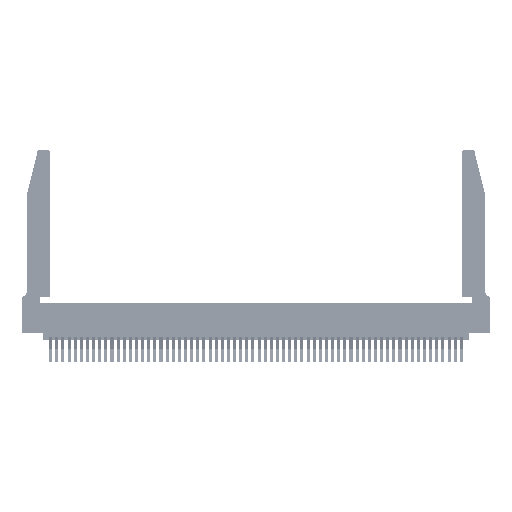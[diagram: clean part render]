
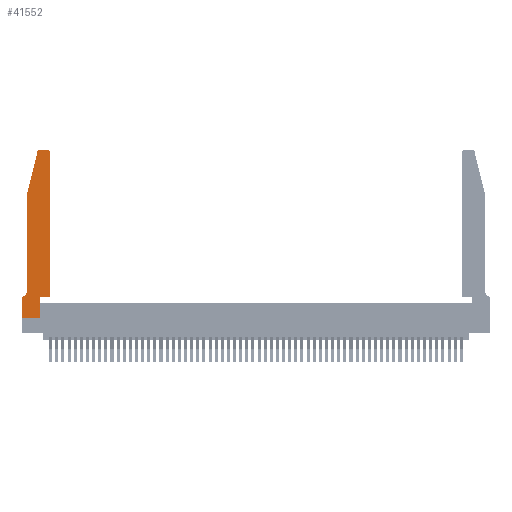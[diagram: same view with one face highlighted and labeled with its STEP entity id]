
A CAD part, top view. The second image highlights one B-rep face of the part: STEP entity #41552.
In plain terms, the highlighted planar face has unit normal (0, 0, 1).
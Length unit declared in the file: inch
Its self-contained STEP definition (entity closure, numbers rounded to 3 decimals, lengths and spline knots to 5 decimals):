
#506 = ORIENTED_EDGE ( 'NONE', *, *, #52466, .T. ) ;
#1064 = CARTESIAN_POINT ( 'NONE',  ( 0.284, 2.72, 0.37 ) ) ;
#1085 = AXIS2_PLACEMENT_3D ( 'NONE', #30913, #9419, #38880 ) ;
#1882 = DIRECTION ( 'NONE',  ( 0., -1., 0. ) ) ;
#2867 = VERTEX_POINT ( 'NONE', #22507 ) ;
#3102 = VERTEX_POINT ( 'NONE', #41610 ) ;
#3352 = DIRECTION ( 'NONE',  ( 0., 1., 0. ) ) ;
#3714 = VERTEX_POINT ( 'NONE', #50578 ) ;
#4692 = CARTESIAN_POINT ( 'NONE',  ( 0.4505, 0.35, 0.37 ) ) ;
#4721 = CARTESIAN_POINT ( 'NONE',  ( 0.2605, 2.75, 0.37 ) ) ;
#5341 = DIRECTION ( 'NONE',  ( 0., 0., 1. ) ) ;
#5504 = VECTOR ( 'NONE', #34674, 39.37008 ) ;
#6053 = ORIENTED_EDGE ( 'NONE', *, *, #23268, .T. ) ;
#6073 = CARTESIAN_POINT ( 'NONE',  ( 0.4205, 2.75, 0.37 ) ) ;
#6304 = VERTEX_POINT ( 'NONE', #43441 ) ;
#6562 = LINE ( 'NONE', #4721, #50968 ) ;
#6827 = LINE ( 'NONE', #18709, #5504 ) ;
#8562 = VERTEX_POINT ( 'NONE', #16446 ) ;
#9251 = LINE ( 'NONE', #15184, #30469 ) ;
#9419 = DIRECTION ( 'NONE',  ( 0., 0., 1. ) ) ;
#9603 = VERTEX_POINT ( 'NONE', #38207 ) ;
#9694 = EDGE_CURVE ( 'NONE', #6304, #2867, #43880, .T. ) ;
#10187 = CARTESIAN_POINT ( 'NONE',  ( 0., 0., 0.37 ) ) ;
#10764 = EDGE_CURVE ( 'NONE', #15551, #9603, #6562, .T. ) ;
#10932 = CIRCLE ( 'NONE', #53073, 0.07 ) ;
#10985 = DIRECTION ( 'NONE',  ( 1., 0., 0. ) ) ;
#11392 = DIRECTION ( 'NONE',  ( -1., 0., 0. ) ) ;
#11738 = CARTESIAN_POINT ( 'NONE',  ( 0.0055, 0.42, 0.37 ) ) ;
#12005 = VECTOR ( 'NONE', #18521, 39.37008 ) ;
#12232 = ORIENTED_EDGE ( 'NONE', *, *, #9694, .T. ) ;
#13826 = ORIENTED_EDGE ( 'NONE', *, *, #10764, .T. ) ;
#13906 = EDGE_CURVE ( 'NONE', #50789, #3714, #10932, .T. ) ;
#14759 = ORIENTED_EDGE ( 'NONE', *, *, #17824, .T. ) ;
#14762 = FACE_OUTER_BOUND ( 'NONE', #15753, .T. ) ;
#14810 = CARTESIAN_POINT ( 'NONE',  ( 0.0755, 0.42, 0.37 ) ) ;
#15184 = CARTESIAN_POINT ( 'NONE',  ( 0.2865, 0.35, 0.37 ) ) ;
#15551 = VERTEX_POINT ( 'NONE', #6073 ) ;
#15753 = EDGE_LOOP ( 'NONE', ( #13826, #19654, #27591, #53457, #26829, #46056, #14759, #12232, #38627, #6053, #506, #33454 ) ) ;
#15930 = VECTOR ( 'NONE', #34876, 39.37008 ) ;
#16446 = CARTESIAN_POINT ( 'NONE',  ( 0.25487, 2.72718, 0.37 ) ) ;
#16465 = AXIS2_PLACEMENT_3D ( 'NONE', #1064, #5341, #35334 ) ;
#17552 = PLANE ( 'NONE',  #1085 ) ;
#17824 = EDGE_CURVE ( 'NONE', #42799, #6304, #25802, .T. ) ;
#17962 = VECTOR ( 'NONE', #1882, 39.37008 ) ;
#18521 = DIRECTION ( 'NONE',  ( 1., 0., 0. ) ) ;
#18709 = CARTESIAN_POINT ( 'NONE',  ( 0.0755, 0.35, 0.37 ) ) ;
#19654 = ORIENTED_EDGE ( 'NONE', *, *, #48358, .T. ) ;
#21516 = VECTOR ( 'NONE', #36218, 39.37008 ) ;
#22507 = CARTESIAN_POINT ( 'NONE',  ( 0.2865, 0., 0.37 ) ) ;
#23268 = EDGE_CURVE ( 'NONE', #35293, #23923, #53949, .T. ) ;
#23913 = EDGE_CURVE ( 'NONE', #3102, #15551, #49177, .T. ) ;
#23923 = VERTEX_POINT ( 'NONE', #40965 ) ;
#25242 = LINE ( 'NONE', #4692, #15930 ) ;
#25802 = LINE ( 'NONE', #28929, #41071 ) ;
#26232 = EDGE_CURVE ( 'NONE', #36796, #50789, #54436, .T. ) ;
#26829 = ORIENTED_EDGE ( 'NONE', *, *, #13906, .T. ) ;
#27591 = ORIENTED_EDGE ( 'NONE', *, *, #48375, .T. ) ;
#28174 = DIRECTION ( 'NONE',  ( 0., 0., 1. ) ) ;
#28278 = DIRECTION ( 'NONE',  ( 0., 0., -1. ) ) ;
#28599 = AXIS2_PLACEMENT_3D ( 'NONE', #49247, #28174, #36506 ) ;
#28660 = CARTESIAN_POINT ( 'NONE',  ( 0.2865, 0.35, 0.37 ) ) ;
#28929 = CARTESIAN_POINT ( 'NONE',  ( 0., 0., 0.37 ) ) ;
#30469 = VECTOR ( 'NONE', #3352, 39.37008 ) ;
#30913 = CARTESIAN_POINT ( 'NONE',  ( 0., 0.35, 0.37 ) ) ;
#32322 = CARTESIAN_POINT ( 'NONE',  ( 0.4505, 0.35, 0.37 ) ) ;
#32751 = VECTOR ( 'NONE', #10985, 39.37008 ) ;
#32819 = LINE ( 'NONE', #38860, #21516 ) ;
#33454 = ORIENTED_EDGE ( 'NONE', *, *, #23913, .T. ) ;
#34516 = CARTESIAN_POINT ( 'NONE',  ( 0., 0.35, 0.37 ) ) ;
#34674 = DIRECTION ( 'NONE',  ( -1., 0., 0. ) ) ;
#34876 = DIRECTION ( 'NONE',  ( 0., 1., 0. ) ) ;
#35293 = VERTEX_POINT ( 'NONE', #28660 ) ;
#35334 = DIRECTION ( 'NONE',  ( 1., 0., 0. ) ) ;
#36218 = DIRECTION ( 'NONE',  ( -0.239, -0.971, 0. ) ) ;
#36506 = DIRECTION ( 'NONE',  ( 1., 0., 0. ) ) ;
#36528 = CARTESIAN_POINT ( 'NONE',  ( 0.0755, 2., 0.37 ) ) ;
#36796 = VERTEX_POINT ( 'NONE', #50878 ) ;
#38207 = CARTESIAN_POINT ( 'NONE',  ( 0.284, 2.75, 0.37 ) ) ;
#38627 = ORIENTED_EDGE ( 'NONE', *, *, #53256, .T. ) ;
#38860 = CARTESIAN_POINT ( 'NONE',  ( 0.0755, 2., 0.37 ) ) ;
#38880 = DIRECTION ( 'NONE',  ( 1., 0., 0. ) ) ;
#40965 = CARTESIAN_POINT ( 'NONE',  ( 0.4505, 0.35, 0.37 ) ) ;
#41071 = VECTOR ( 'NONE', #41730, 39.37008 ) ;
#41552 = ADVANCED_FACE ( 'NONE', ( #14762 ), #17552, .T. ) ;
#41610 = CARTESIAN_POINT ( 'NONE',  ( 0.4505, 2.72, 0.37 ) ) ;
#41730 = DIRECTION ( 'NONE',  ( 0., -1., 0. ) ) ;
#42128 = CIRCLE ( 'NONE', #16465, 0.03 ) ;
#42799 = VERTEX_POINT ( 'NONE', #34516 ) ;
#43441 = CARTESIAN_POINT ( 'NONE',  ( 0., 0., 0.37 ) ) ;
#43880 = LINE ( 'NONE', #10187, #12005 ) ;
#46056 = ORIENTED_EDGE ( 'NONE', *, *, #49584, .T. ) ;
#48358 = EDGE_CURVE ( 'NONE', #9603, #8562, #42128, .T. ) ;
#48375 = EDGE_CURVE ( 'NONE', #8562, #36796, #32819, .T. ) ;
#49177 = CIRCLE ( 'NONE', #28599, 0.03 ) ;
#49247 = CARTESIAN_POINT ( 'NONE',  ( 0.4205, 2.72, 0.37 ) ) ;
#49584 = EDGE_CURVE ( 'NONE', #3714, #42799, #6827, .T. ) ;
#50578 = CARTESIAN_POINT ( 'NONE',  ( 0.0055, 0.35, 0.37 ) ) ;
#50789 = VERTEX_POINT ( 'NONE', #14810 ) ;
#50878 = CARTESIAN_POINT ( 'NONE',  ( 0.0755, 2., 0.37 ) ) ;
#50968 = VECTOR ( 'NONE', #51171, 39.37008 ) ;
#51171 = DIRECTION ( 'NONE',  ( -1., 0., 0. ) ) ;
#52466 = EDGE_CURVE ( 'NONE', #23923, #3102, #25242, .T. ) ;
#53073 = AXIS2_PLACEMENT_3D ( 'NONE', #11738, #28278, #11392 ) ;
#53256 = EDGE_CURVE ( 'NONE', #2867, #35293, #9251, .T. ) ;
#53457 = ORIENTED_EDGE ( 'NONE', *, *, #26232, .T. ) ;
#53949 = LINE ( 'NONE', #32322, #32751 ) ;
#54436 = LINE ( 'NONE', #36528, #17962 ) ;
